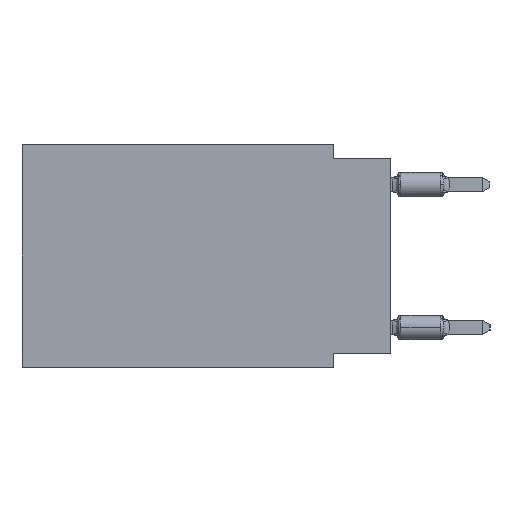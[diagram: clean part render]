
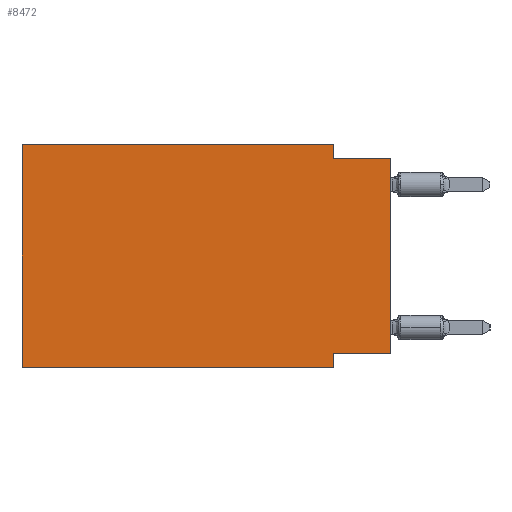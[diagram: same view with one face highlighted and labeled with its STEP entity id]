
A CAD part, left-side view. The second image highlights one B-rep face of the part: STEP entity #8472.
In plain terms, the highlighted planar face has unit normal (-1, 0, 0).
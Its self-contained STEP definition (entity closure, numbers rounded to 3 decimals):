
#915 = DIRECTION ( 'NONE',  ( 1., 0., 0. ) ) ;
#957 = CARTESIAN_POINT ( 'NONE',  ( 0., 16.383, -9.906 ) ) ;
#1187 = EDGE_CURVE ( 'NONE', #17176, #17320, #9095, .T. ) ;
#1774 = CARTESIAN_POINT ( 'NONE',  ( 0., 16.383, 0. ) ) ;
#2354 = VERTEX_POINT ( 'NONE', #4947 ) ;
#2841 = ORIENTED_EDGE ( 'NONE', *, *, #9288, .F. ) ;
#3167 = CARTESIAN_POINT ( 'NONE',  ( 0., 0., -9.271 ) ) ;
#3492 = VERTEX_POINT ( 'NONE', #16974 ) ;
#3593 = CARTESIAN_POINT ( 'NONE',  ( 0., 0., -0.635 ) ) ;
#3822 = DIRECTION ( 'NONE',  ( 0., 0., -1. ) ) ;
#4947 = CARTESIAN_POINT ( 'NONE',  ( 0., 0., -9.271 ) ) ;
#4961 = EDGE_CURVE ( 'NONE', #11337, #26795, #26931, .T. ) ;
#5439 = ORIENTED_EDGE ( 'NONE', *, *, #13709, .T. ) ;
#7850 = VECTOR ( 'NONE', #21764, 1000. ) ;
#8426 = VERTEX_POINT ( 'NONE', #26034 ) ;
#8472 = ADVANCED_FACE ( 'NONE', ( #13635 ), #14307, .F. ) ;
#8592 = VECTOR ( 'NONE', #33158, 1000. ) ;
#8648 = LINE ( 'NONE', #14311, #9250 ) ;
#8937 = LINE ( 'NONE', #27497, #8592 ) ;
#9095 = LINE ( 'NONE', #3593, #31568 ) ;
#9250 = VECTOR ( 'NONE', #29955, 1000. ) ;
#9288 = EDGE_CURVE ( 'NONE', #8426, #19352, #9843, .T. ) ;
#9843 = LINE ( 'NONE', #1774, #30287 ) ;
#11298 = CARTESIAN_POINT ( 'NONE',  ( 0., 2.54, -9.906 ) ) ;
#11337 = VERTEX_POINT ( 'NONE', #33372 ) ;
#12600 = ORIENTED_EDGE ( 'NONE', *, *, #27206, .T. ) ;
#12973 = EDGE_CURVE ( 'NONE', #3492, #8426, #8937, .T. ) ;
#13635 = FACE_OUTER_BOUND ( 'NONE', #23638, .T. ) ;
#13709 = EDGE_CURVE ( 'NONE', #3492, #26795, #30165, .T. ) ;
#13999 = AXIS2_PLACEMENT_3D ( 'NONE', #29785, #915, #3822 ) ;
#14307 = PLANE ( 'NONE',  #13999 ) ;
#14311 = CARTESIAN_POINT ( 'NONE',  ( 0., 2.54, 0. ) ) ;
#14676 = ORIENTED_EDGE ( 'NONE', *, *, #1187, .F. ) ;
#15519 = ORIENTED_EDGE ( 'NONE', *, *, #16415, .F. ) ;
#16177 = ORIENTED_EDGE ( 'NONE', *, *, #27414, .F. ) ;
#16415 = EDGE_CURVE ( 'NONE', #2354, #11337, #29458, .T. ) ;
#16974 = CARTESIAN_POINT ( 'NONE',  ( 0., 16.383, -9.906 ) ) ;
#17176 = VERTEX_POINT ( 'NONE', #28847 ) ;
#17320 = VERTEX_POINT ( 'NONE', #19340 ) ;
#18488 = VECTOR ( 'NONE', #30341, 1000. ) ;
#19340 = CARTESIAN_POINT ( 'NONE',  ( 0., 0., -0.635 ) ) ;
#19352 = VERTEX_POINT ( 'NONE', #32721 ) ;
#21020 = ORIENTED_EDGE ( 'NONE', *, *, #4961, .F. ) ;
#21764 = DIRECTION ( 'NONE',  ( 0., 0., -1. ) ) ;
#22068 = CARTESIAN_POINT ( 'NONE',  ( 0., 2.54, -9.906 ) ) ;
#23638 = EDGE_LOOP ( 'NONE', ( #12600, #14676, #16177, #2841, #24465, #5439, #21020, #15519 ) ) ;
#24465 = ORIENTED_EDGE ( 'NONE', *, *, #12973, .F. ) ;
#25067 = DIRECTION ( 'NONE',  ( 0., -1., 0. ) ) ;
#26034 = CARTESIAN_POINT ( 'NONE',  ( 0., 16.383, 0. ) ) ;
#26795 = VERTEX_POINT ( 'NONE', #22068 ) ;
#26931 = LINE ( 'NONE', #11298, #7850 ) ;
#27049 = DIRECTION ( 'NONE',  ( 0., 1., 0. ) ) ;
#27206 = EDGE_CURVE ( 'NONE', #2354, #17320, #28267, .T. ) ;
#27381 = VECTOR ( 'NONE', #27049, 1000. ) ;
#27414 = EDGE_CURVE ( 'NONE', #19352, #17176, #8648, .T. ) ;
#27497 = CARTESIAN_POINT ( 'NONE',  ( 0., 16.383, 0. ) ) ;
#28267 = LINE ( 'NONE', #33777, #29784 ) ;
#28847 = CARTESIAN_POINT ( 'NONE',  ( 0., 2.54, -0.635 ) ) ;
#29458 = LINE ( 'NONE', #3167, #27381 ) ;
#29784 = VECTOR ( 'NONE', #33258, 1000. ) ;
#29785 = CARTESIAN_POINT ( 'NONE',  ( 0., 16.383, 0. ) ) ;
#29955 = DIRECTION ( 'NONE',  ( 0., 0., -1. ) ) ;
#30165 = LINE ( 'NONE', #957, #18488 ) ;
#30287 = VECTOR ( 'NONE', #32716, 1000. ) ;
#30341 = DIRECTION ( 'NONE',  ( 0., -1., 0. ) ) ;
#31568 = VECTOR ( 'NONE', #25067, 1000. ) ;
#32716 = DIRECTION ( 'NONE',  ( 0., -1., 0. ) ) ;
#32721 = CARTESIAN_POINT ( 'NONE',  ( 0., 2.54, 0. ) ) ;
#33158 = DIRECTION ( 'NONE',  ( 0., 0., 1. ) ) ;
#33258 = DIRECTION ( 'NONE',  ( 0., 0., 1. ) ) ;
#33372 = CARTESIAN_POINT ( 'NONE',  ( 0., 2.54, -9.271 ) ) ;
#33777 = CARTESIAN_POINT ( 'NONE',  ( 0., 0., 0. ) ) ;
